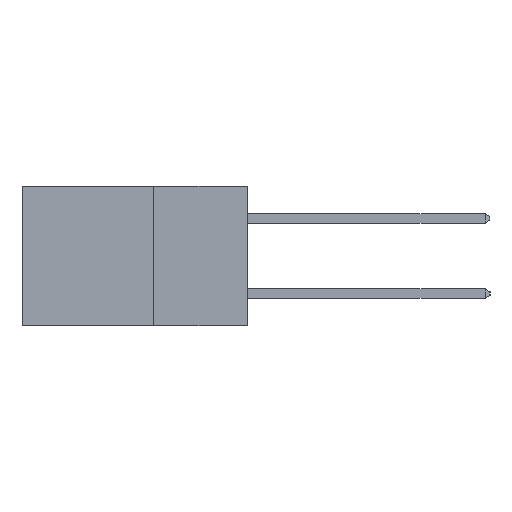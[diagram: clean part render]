
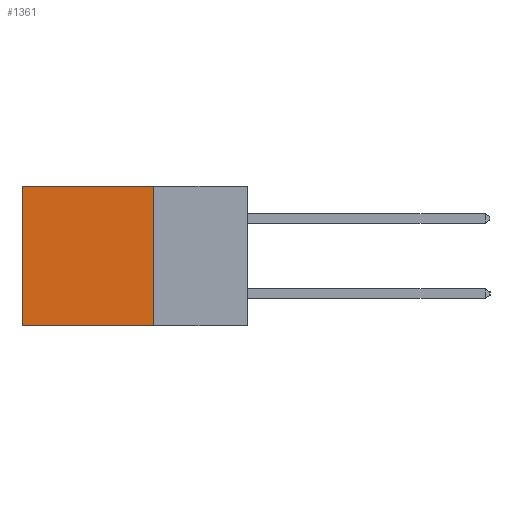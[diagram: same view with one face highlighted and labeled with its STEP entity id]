
A CAD part, left-side view. The second image highlights one B-rep face of the part: STEP entity #1361.
In plain terms, the highlighted planar face has unit normal (-1, 0, 0).
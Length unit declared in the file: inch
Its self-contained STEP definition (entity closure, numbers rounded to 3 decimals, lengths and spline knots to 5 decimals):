
#258 = LINE ( 'NONE', #5725, #10740 ) ;
#623 = VERTEX_POINT ( 'NONE', #4683 ) ;
#649 = LINE ( 'NONE', #8391, #11075 ) ;
#1054 = LINE ( 'NONE', #4584, #2172 ) ;
#1102 = ORIENTED_EDGE ( 'NONE', *, *, #7099, .T. ) ;
#1361 = ADVANCED_FACE ( 'NONE', ( #10101 ), #1517, .F. ) ;
#1517 = PLANE ( 'NONE',  #3151 ) ;
#2172 = VECTOR ( 'NONE', #4739, 39.37008 ) ;
#2929 = CARTESIAN_POINT ( 'NONE',  ( 0.2615, 0.25, -0.37 ) ) ;
#3151 = AXIS2_PLACEMENT_3D ( 'NONE', #7893, #7807, #12102 ) ;
#4403 = VECTOR ( 'NONE', #12000, 39.37008 ) ;
#4418 = EDGE_CURVE ( 'NONE', #6666, #8576, #258, .T. ) ;
#4584 = CARTESIAN_POINT ( 'NONE',  ( 0.2615, 0.6, -0.37 ) ) ;
#4648 = EDGE_CURVE ( 'NONE', #6946, #8576, #1054, .T. ) ;
#4683 = CARTESIAN_POINT ( 'NONE',  ( 0.2615, 0.25, 0. ) ) ;
#4739 = DIRECTION ( 'NONE',  ( 0., 0., -1. ) ) ;
#5394 = DIRECTION ( 'NONE',  ( 0., 0., -1. ) ) ;
#5593 = DIRECTION ( 'NONE',  ( 0., 1., 0. ) ) ;
#5725 = CARTESIAN_POINT ( 'NONE',  ( 0.2615, 0.25, -0.37 ) ) ;
#6256 = ORIENTED_EDGE ( 'NONE', *, *, #4648, .T. ) ;
#6666 = VERTEX_POINT ( 'NONE', #2929 ) ;
#6946 = VERTEX_POINT ( 'NONE', #12604 ) ;
#7099 = EDGE_CURVE ( 'NONE', #623, #6946, #11609, .T. ) ;
#7807 = DIRECTION ( 'NONE',  ( 1., 0., 0. ) ) ;
#7893 = CARTESIAN_POINT ( 'NONE',  ( 0.2615, 0.25, -0.37 ) ) ;
#8120 = EDGE_LOOP ( 'NONE', ( #6256, #11167, #11428, #1102 ) ) ;
#8391 = CARTESIAN_POINT ( 'NONE',  ( 0.2615, 0.25, -0.37 ) ) ;
#8576 = VERTEX_POINT ( 'NONE', #9176 ) ;
#8764 = EDGE_CURVE ( 'NONE', #623, #6666, #649, .T. ) ;
#9176 = CARTESIAN_POINT ( 'NONE',  ( 0.2615, 0.6, -0.37 ) ) ;
#10101 = FACE_OUTER_BOUND ( 'NONE', #8120, .T. ) ;
#10740 = VECTOR ( 'NONE', #5593, 39.37008 ) ;
#11075 = VECTOR ( 'NONE', #5394, 39.37008 ) ;
#11167 = ORIENTED_EDGE ( 'NONE', *, *, #4418, .F. ) ;
#11428 = ORIENTED_EDGE ( 'NONE', *, *, #8764, .F. ) ;
#11609 = LINE ( 'NONE', #12057, #4403 ) ;
#12000 = DIRECTION ( 'NONE',  ( 0., 1., 0. ) ) ;
#12057 = CARTESIAN_POINT ( 'NONE',  ( 0.2615, 0.25, 0. ) ) ;
#12102 = DIRECTION ( 'NONE',  ( 0., 0., -1. ) ) ;
#12604 = CARTESIAN_POINT ( 'NONE',  ( 0.2615, 0.6, 0. ) ) ;
